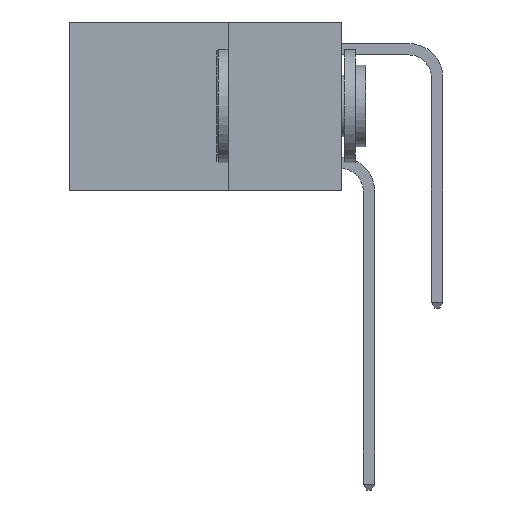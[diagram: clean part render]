
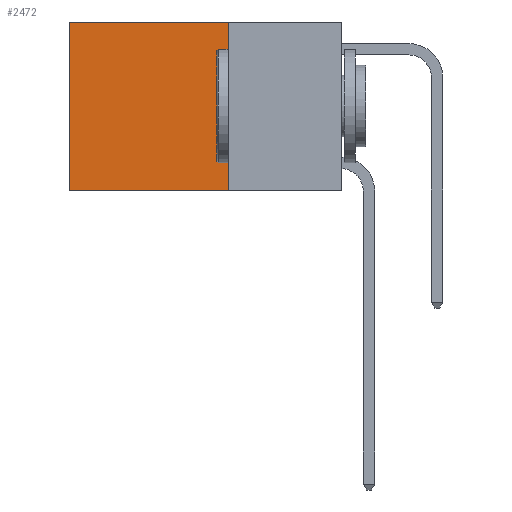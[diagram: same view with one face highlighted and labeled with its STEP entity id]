
A CAD part, left-side view. The second image highlights one B-rep face of the part: STEP entity #2472.
In plain terms, the highlighted planar face has unit normal (-1, 0, 0).
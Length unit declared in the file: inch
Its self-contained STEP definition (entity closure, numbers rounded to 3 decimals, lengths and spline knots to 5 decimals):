
#84 = ORIENTED_EDGE ( 'NONE', *, *, #3778, .T. ) ;
#294 = LINE ( 'NONE', #4137, #10635 ) ;
#328 = EDGE_LOOP ( 'NONE', ( #84, #5596, #8176, #10774 ) ) ;
#393 = DIRECTION ( 'NONE',  ( 0., 0., -1. ) ) ;
#490 = VERTEX_POINT ( 'NONE', #3436 ) ;
#1065 = EDGE_CURVE ( 'NONE', #10803, #2971, #2331, .T. ) ;
#1102 = CARTESIAN_POINT ( 'NONE',  ( 0.2625, 0.25, -0.37 ) ) ;
#1287 = DIRECTION ( 'NONE',  ( 0., 1., 0. ) ) ;
#1370 = VERTEX_POINT ( 'NONE', #3900 ) ;
#2331 = LINE ( 'NONE', #1102, #10387 ) ;
#2472 = ADVANCED_FACE ( 'NONE', ( #11619 ), #11066, .F. ) ;
#2971 = VERTEX_POINT ( 'NONE', #4095 ) ;
#3402 = VECTOR ( 'NONE', #10899, 39.37008 ) ;
#3436 = CARTESIAN_POINT ( 'NONE',  ( 0.2625, 0.25, 0. ) ) ;
#3666 = CARTESIAN_POINT ( 'NONE',  ( 0.2625, 0.25, 0. ) ) ;
#3778 = EDGE_CURVE ( 'NONE', #1370, #2971, #11100, .T. ) ;
#3900 = CARTESIAN_POINT ( 'NONE',  ( 0.2625, 0.6, 0. ) ) ;
#4095 = CARTESIAN_POINT ( 'NONE',  ( 0.2625, 0.6, -0.37 ) ) ;
#4137 = CARTESIAN_POINT ( 'NONE',  ( 0.2625, 0.25, 0. ) ) ;
#4592 = LINE ( 'NONE', #3666, #7448 ) ;
#4976 = CARTESIAN_POINT ( 'NONE',  ( 0.2625, 0.25, -0.37 ) ) ;
#5116 = DIRECTION ( 'NONE',  ( 0., 1., 0. ) ) ;
#5120 = EDGE_CURVE ( 'NONE', #490, #10803, #4592, .T. ) ;
#5577 = EDGE_CURVE ( 'NONE', #490, #1370, #294, .T. ) ;
#5596 = ORIENTED_EDGE ( 'NONE', *, *, #1065, .F. ) ;
#6072 = AXIS2_PLACEMENT_3D ( 'NONE', #8138, #12079, #6233 ) ;
#6233 = DIRECTION ( 'NONE',  ( 0., 0., -1. ) ) ;
#7448 = VECTOR ( 'NONE', #393, 39.37008 ) ;
#8138 = CARTESIAN_POINT ( 'NONE',  ( 0.2625, 0.25, 0. ) ) ;
#8176 = ORIENTED_EDGE ( 'NONE', *, *, #5120, .F. ) ;
#10387 = VECTOR ( 'NONE', #1287, 39.37008 ) ;
#10635 = VECTOR ( 'NONE', #5116, 39.37008 ) ;
#10774 = ORIENTED_EDGE ( 'NONE', *, *, #5577, .T. ) ;
#10803 = VERTEX_POINT ( 'NONE', #4976 ) ;
#10899 = DIRECTION ( 'NONE',  ( 0., 0., -1. ) ) ;
#11066 = PLANE ( 'NONE',  #6072 ) ;
#11100 = LINE ( 'NONE', #11904, #3402 ) ;
#11619 = FACE_OUTER_BOUND ( 'NONE', #328, .T. ) ;
#11904 = CARTESIAN_POINT ( 'NONE',  ( 0.2625, 0.6, 0. ) ) ;
#12079 = DIRECTION ( 'NONE',  ( 1., 0., 0. ) ) ;
